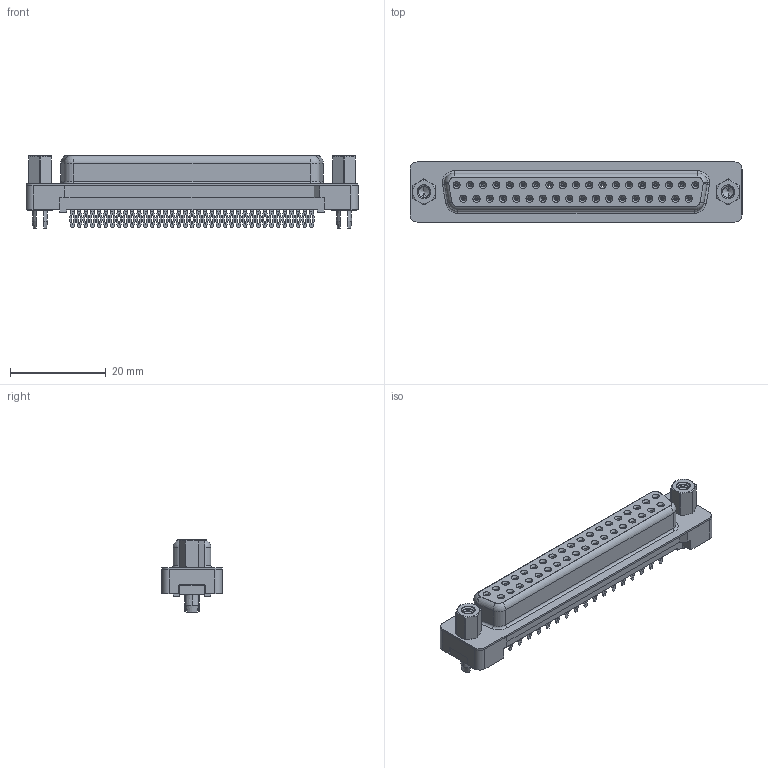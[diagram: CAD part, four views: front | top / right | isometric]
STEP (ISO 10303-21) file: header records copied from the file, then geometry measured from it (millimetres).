
FILE_DESCRIPTION (( 'STEP AP203' ), '1' );
FILE_NAME ('628-037-626-017.STEP', '2020-07-16T00:58:37', ( '' ), ( '' ), 'SwSTEP 2.0', 'SolidWorks 2020', '' );
FILE_SCHEMA (( 'CONFIG_CONTROL_DESIGN' ));
Length unit declared in the file: millimetre
Products named in the file (7): 628 Plastic Body Housing_37 Contacts; 628 4-40 Hex Standoff; 628 PB 4-40 Threaded Rivet with Boardlock; 628 PB Contact Row 1_26; 628 PB Contact Row 2_26; 628-037-626-017; 628 PB Shell_37 Contacts
Assembly tree (43 placements, depth 2):
  628-037-626-017
    628 Plastic Body Housing_37 Contacts
    628 PB Shell_37 Contacts
    628 PB Contact Row 1_26  x19
    628 PB Contact Row 2_26  x18
    628 4-40 Hex Standoff  x2
    628 PB 4-40 Threaded Rivet with Boardlock  x2
Bounding box: 69.32 x 12.55 x 15.05 mm (x, y, z)
Volume: 4471.4 mm3; surface area: 12096.9 mm2
Topology: 43 solids, 43 shells, 3717 faces, 9103 edges, 5522 vertices
Faces by surface type: plane 1500, cylinder 910, bspline 832, torus 248, cone 227
Entity records: 29558 total; most frequent: CARTESIAN_POINT 9562, ORIENTED_EDGE 3832, DIRECTION 3682, EDGE_CURVE 1916, AXIS2_PLACEMENT_3D 1268, VERTEX_POINT 1206, VECTOR 1146, LINE 1146
